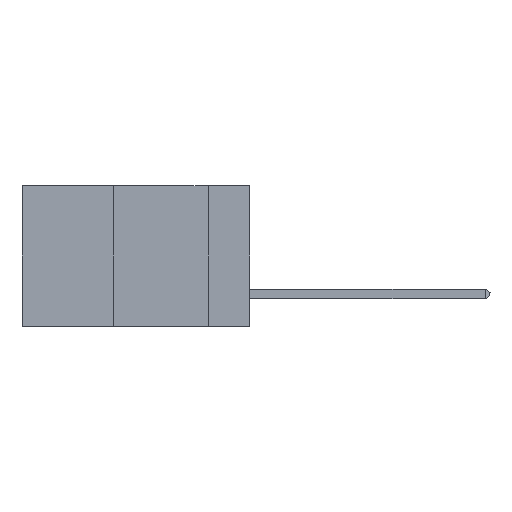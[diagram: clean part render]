
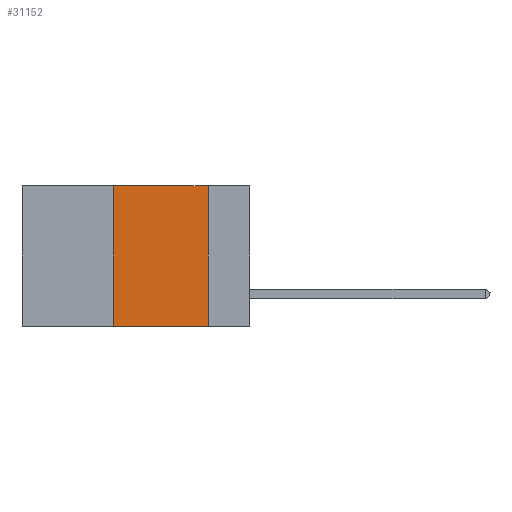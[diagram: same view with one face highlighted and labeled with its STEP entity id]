
A CAD part, left-side view. The second image highlights one B-rep face of the part: STEP entity #31152.
In plain terms, the highlighted planar face has unit normal (-1, 0, 0).
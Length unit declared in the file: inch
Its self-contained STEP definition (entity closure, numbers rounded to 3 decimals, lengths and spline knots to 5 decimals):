
#514 = LINE ( 'NONE', #12417, #34293 ) ;
#654 = CARTESIAN_POINT ( 'NONE',  ( 0., 0.36, 0. ) ) ;
#966 = VECTOR ( 'NONE', #18750, 39.37008 ) ;
#1078 = ORIENTED_EDGE ( 'NONE', *, *, #11196, .F. ) ;
#1113 = DIRECTION ( 'NONE',  ( 0., -1., 0. ) ) ;
#2080 = EDGE_LOOP ( 'NONE', ( #1078, #13078, #9105, #10137 ) ) ;
#2349 = VECTOR ( 'NONE', #29502, 39.37008 ) ;
#3728 = VERTEX_POINT ( 'NONE', #29028 ) ;
#6806 = VERTEX_POINT ( 'NONE', #26299 ) ;
#8172 = PLANE ( 'NONE',  #36838 ) ;
#8463 = CARTESIAN_POINT ( 'NONE',  ( 0., 0.6, 0. ) ) ;
#9105 = ORIENTED_EDGE ( 'NONE', *, *, #27700, .F. ) ;
#10137 = ORIENTED_EDGE ( 'NONE', *, *, #33934, .T. ) ;
#11196 = EDGE_CURVE ( 'NONE', #21890, #6806, #22300, .T. ) ;
#12417 = CARTESIAN_POINT ( 'NONE',  ( 0., 0.6, 0. ) ) ;
#12649 = CARTESIAN_POINT ( 'NONE',  ( 0., 0.11, 0. ) ) ;
#13078 = ORIENTED_EDGE ( 'NONE', *, *, #37170, .F. ) ;
#13644 = DIRECTION ( 'NONE',  ( 0., 0., -1. ) ) ;
#13736 = LINE ( 'NONE', #31798, #19206 ) ;
#14720 = LINE ( 'NONE', #654, #2349 ) ;
#18750 = DIRECTION ( 'NONE',  ( 0., 0., -1. ) ) ;
#18798 = CARTESIAN_POINT ( 'NONE',  ( 0., 0.11, 0. ) ) ;
#19206 = VECTOR ( 'NONE', #1113, 39.37008 ) ;
#19829 = DIRECTION ( 'NONE',  ( 0., -1., 0. ) ) ;
#21890 = VERTEX_POINT ( 'NONE', #18798 ) ;
#22300 = LINE ( 'NONE', #12649, #966 ) ;
#22848 = FACE_OUTER_BOUND ( 'NONE', #2080, .T. ) ;
#24791 = DIRECTION ( 'NONE',  ( 1., 0., 0. ) ) ;
#26299 = CARTESIAN_POINT ( 'NONE',  ( 0., 0.11, -0.37 ) ) ;
#27700 = EDGE_CURVE ( 'NONE', #30662, #3728, #14720, .T. ) ;
#28915 = CARTESIAN_POINT ( 'NONE',  ( 0., 0.36, -0.37 ) ) ;
#29028 = CARTESIAN_POINT ( 'NONE',  ( 0., 0.36, 0. ) ) ;
#29502 = DIRECTION ( 'NONE',  ( 0., 0., 1. ) ) ;
#30662 = VERTEX_POINT ( 'NONE', #28915 ) ;
#31152 = ADVANCED_FACE ( 'NONE', ( #22848 ), #8172, .F. ) ;
#31798 = CARTESIAN_POINT ( 'NONE',  ( 0., 0.6, -0.37 ) ) ;
#33934 = EDGE_CURVE ( 'NONE', #30662, #6806, #13736, .T. ) ;
#34293 = VECTOR ( 'NONE', #19829, 39.37008 ) ;
#36838 = AXIS2_PLACEMENT_3D ( 'NONE', #8463, #24791, #13644 ) ;
#37170 = EDGE_CURVE ( 'NONE', #3728, #21890, #514, .T. ) ;
